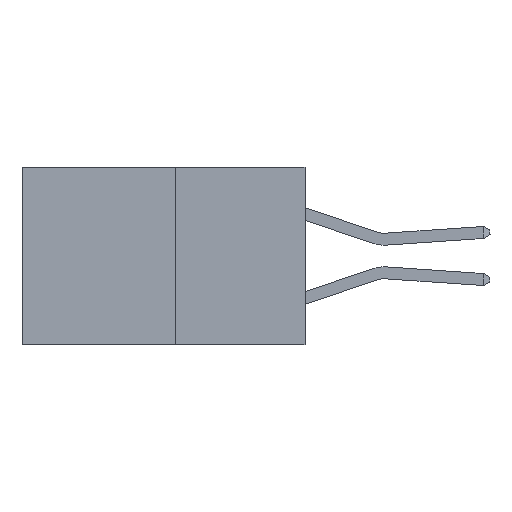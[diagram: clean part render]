
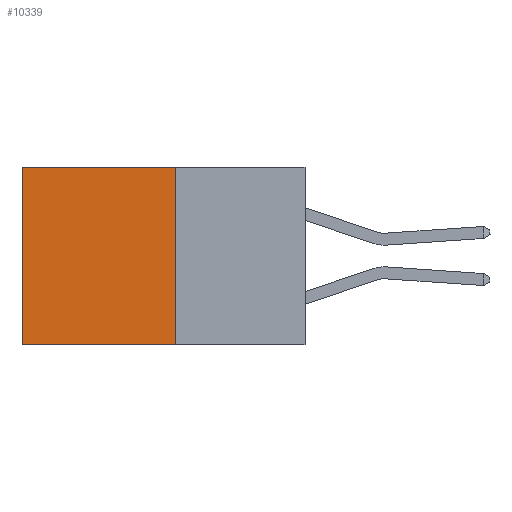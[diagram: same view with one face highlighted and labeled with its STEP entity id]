
A CAD part, left-side view. The second image highlights one B-rep face of the part: STEP entity #10339.
In plain terms, the highlighted planar face has unit normal (-1, 0, 0).
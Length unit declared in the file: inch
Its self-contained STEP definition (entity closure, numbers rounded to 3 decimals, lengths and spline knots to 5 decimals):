
#123 = CARTESIAN_POINT ( 'NONE',  ( 0.277, 0.27, 0. ) ) ;
#609 = LINE ( 'NONE', #4888, #3597 ) ;
#976 = VECTOR ( 'NONE', #9743, 39.37008 ) ;
#1267 = EDGE_LOOP ( 'NONE', ( #13333, #9103, #7727, #2967 ) ) ;
#1376 = LINE ( 'NONE', #8444, #976 ) ;
#1401 = CARTESIAN_POINT ( 'NONE',  ( 0.277, 0.27, 0. ) ) ;
#1932 = CARTESIAN_POINT ( 'NONE',  ( 0.277, 0.59, -0.37 ) ) ;
#2398 = CARTESIAN_POINT ( 'NONE',  ( 0.277, 0.27, -0.37 ) ) ;
#2967 = ORIENTED_EDGE ( 'NONE', *, *, #13750, .T. ) ;
#3108 = EDGE_CURVE ( 'NONE', #6749, #9947, #8903, .T. ) ;
#3200 = EDGE_CURVE ( 'NONE', #9947, #11147, #1376, .T. ) ;
#3597 = VECTOR ( 'NONE', #12352, 39.37008 ) ;
#3702 = VERTEX_POINT ( 'NONE', #7531 ) ;
#4296 = CARTESIAN_POINT ( 'NONE',  ( 0.277, 0.27, -0.37 ) ) ;
#4888 = CARTESIAN_POINT ( 'NONE',  ( 0.277, 0.59, -0.37 ) ) ;
#4956 = DIRECTION ( 'NONE',  ( 1., 0., 0. ) ) ;
#4977 = DIRECTION ( 'NONE',  ( 0., 0., -1. ) ) ;
#6050 = CARTESIAN_POINT ( 'NONE',  ( 0.277, 0.27, -0.37 ) ) ;
#6491 = DIRECTION ( 'NONE',  ( 0., 1., 0. ) ) ;
#6749 = VERTEX_POINT ( 'NONE', #1401 ) ;
#7531 = CARTESIAN_POINT ( 'NONE',  ( 0.277, 0.59, 0. ) ) ;
#7727 = ORIENTED_EDGE ( 'NONE', *, *, #3108, .F. ) ;
#8171 = FACE_OUTER_BOUND ( 'NONE', #1267, .T. ) ;
#8444 = CARTESIAN_POINT ( 'NONE',  ( 0.277, 0.27, -0.37 ) ) ;
#8678 = PLANE ( 'NONE',  #9645 ) ;
#8903 = LINE ( 'NONE', #6050, #15023 ) ;
#9103 = ORIENTED_EDGE ( 'NONE', *, *, #3200, .F. ) ;
#9645 = AXIS2_PLACEMENT_3D ( 'NONE', #2398, #4956, #13646 ) ;
#9743 = DIRECTION ( 'NONE',  ( 0., 1., 0. ) ) ;
#9947 = VERTEX_POINT ( 'NONE', #4296 ) ;
#10339 = ADVANCED_FACE ( 'NONE', ( #8171 ), #8678, .F. ) ;
#10873 = EDGE_CURVE ( 'NONE', #3702, #11147, #609, .T. ) ;
#11147 = VERTEX_POINT ( 'NONE', #1932 ) ;
#12352 = DIRECTION ( 'NONE',  ( 0., 0., -1. ) ) ;
#13333 = ORIENTED_EDGE ( 'NONE', *, *, #10873, .T. ) ;
#13646 = DIRECTION ( 'NONE',  ( 0., 0., -1. ) ) ;
#13660 = VECTOR ( 'NONE', #6491, 39.37008 ) ;
#13750 = EDGE_CURVE ( 'NONE', #6749, #3702, #14043, .T. ) ;
#14043 = LINE ( 'NONE', #123, #13660 ) ;
#15023 = VECTOR ( 'NONE', #4977, 39.37008 ) ;
